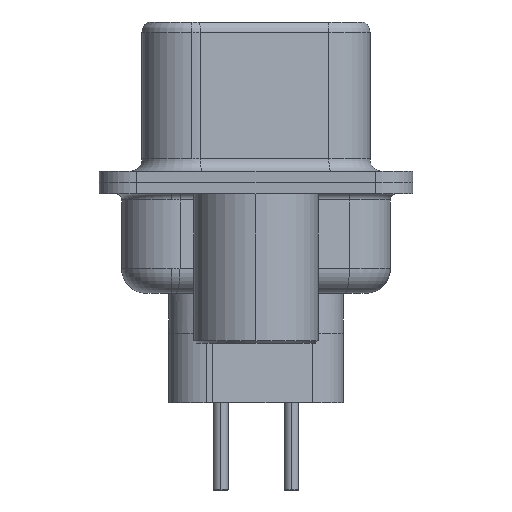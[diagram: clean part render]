
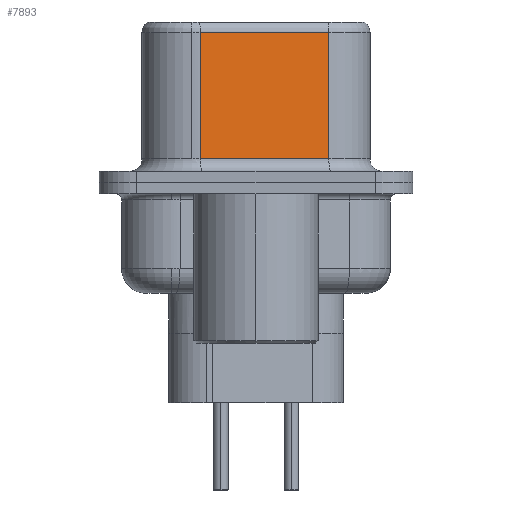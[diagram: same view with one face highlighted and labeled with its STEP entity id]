
A CAD part, left-side view. The second image highlights one B-rep face of the part: STEP entity #7893.
In plain terms, the highlighted planar face has unit normal (-0.985, -0.174, 0).
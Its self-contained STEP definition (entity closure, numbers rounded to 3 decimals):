
#253 = LINE ( 'NONE', #1689, #11228 ) ;
#338 = VERTEX_POINT ( 'NONE', #3338 ) ;
#976 = VERTEX_POINT ( 'NONE', #14528 ) ;
#1689 = CARTESIAN_POINT ( 'NONE',  ( 3.665, 2.233, 6.52 ) ) ;
#1934 = EDGE_LOOP ( 'NONE', ( #11545, #5438, #6260, #6356 ) ) ;
#2610 = DIRECTION ( 'NONE',  ( 0.174, -0.985, 0. ) ) ;
#3338 = CARTESIAN_POINT ( 'NONE',  ( 3.665, 2.233, 0.95 ) ) ;
#3800 = VERTEX_POINT ( 'NONE', #19136 ) ;
#5438 = ORIENTED_EDGE ( 'NONE', *, *, #11373, .T. ) ;
#6260 = ORIENTED_EDGE ( 'NONE', *, *, #17759, .T. ) ;
#6284 = VECTOR ( 'NONE', #2610, 1000. ) ;
#6356 = ORIENTED_EDGE ( 'NONE', *, *, #7105, .T. ) ;
#6501 = DIRECTION ( 'NONE',  ( 0., 0., -1. ) ) ;
#7105 = EDGE_CURVE ( 'NONE', #338, #18773, #19573, .T. ) ;
#7337 = CARTESIAN_POINT ( 'NONE',  ( 4.575, -2.927, 6.52 ) ) ;
#7622 = AXIS2_PLACEMENT_3D ( 'NONE', #7337, #10486, #13549 ) ;
#7633 = DIRECTION ( 'NONE',  ( 0., 0., -1. ) ) ;
#7893 = ADVANCED_FACE ( 'NONE', ( #18232 ), #12116, .F. ) ;
#10171 = CARTESIAN_POINT ( 'NONE',  ( 4.575, -2.927, 6.52 ) ) ;
#10486 = DIRECTION ( 'NONE',  ( 0.985, 0.174, 0. ) ) ;
#10711 = EDGE_CURVE ( 'NONE', #976, #18773, #15060, .T. ) ;
#11228 = VECTOR ( 'NONE', #6501, 1000. ) ;
#11373 = EDGE_CURVE ( 'NONE', #976, #3800, #19376, .T. ) ;
#11545 = ORIENTED_EDGE ( 'NONE', *, *, #10711, .F. ) ;
#12116 = PLANE ( 'NONE',  #7622 ) ;
#13146 = CARTESIAN_POINT ( 'NONE',  ( 4.575, -2.927, 6.02 ) ) ;
#13337 = CARTESIAN_POINT ( 'NONE',  ( 4.575, -2.927, 0.95 ) ) ;
#13467 = VECTOR ( 'NONE', #16107, 1000. ) ;
#13549 = DIRECTION ( 'NONE',  ( -0.174, 0.985, 0. ) ) ;
#14528 = CARTESIAN_POINT ( 'NONE',  ( 4.575, -2.927, 6.02 ) ) ;
#15060 = LINE ( 'NONE', #10171, #16372 ) ;
#16107 = DIRECTION ( 'NONE',  ( -0.174, 0.985, 0. ) ) ;
#16372 = VECTOR ( 'NONE', #7633, 1000. ) ;
#17759 = EDGE_CURVE ( 'NONE', #3800, #338, #253, .T. ) ;
#17852 = CARTESIAN_POINT ( 'NONE',  ( 4.575, -2.927, 0.95 ) ) ;
#18232 = FACE_OUTER_BOUND ( 'NONE', #1934, .T. ) ;
#18773 = VERTEX_POINT ( 'NONE', #17852 ) ;
#19136 = CARTESIAN_POINT ( 'NONE',  ( 3.665, 2.233, 6.02 ) ) ;
#19376 = LINE ( 'NONE', #13146, #13467 ) ;
#19573 = LINE ( 'NONE', #13337, #6284 ) ;
